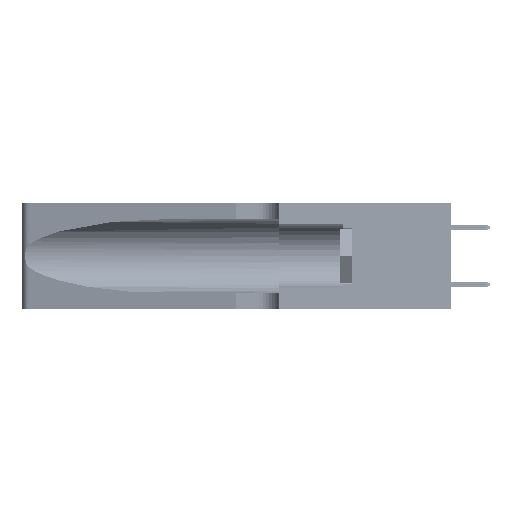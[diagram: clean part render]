
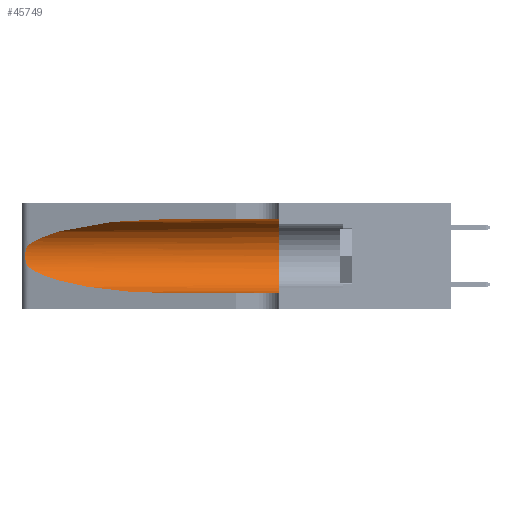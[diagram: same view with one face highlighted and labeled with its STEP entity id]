
A CAD part, left-side view. The second image highlights one B-rep face of the part: STEP entity #45749.
In plain terms, the highlighted cylindrical face has radius 3.308 mm (diameter 6.617 mm), a partial arc.
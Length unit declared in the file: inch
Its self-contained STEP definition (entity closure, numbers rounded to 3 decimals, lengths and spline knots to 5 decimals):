
#365 = CARTESIAN_POINT ( 'NONE',  ( 0.25487, 1.22718, 0.14631 ) ) ;
#1262 = CARTESIAN_POINT ( 'NONE',  ( 0.26075, 1.23896, 0.178 ) ) ;
#1339 = LINE ( 'NONE', #4804, #31778 ) ;
#3054 = CARTESIAN_POINT ( 'NONE',  ( 0.25487, 1.22718, 0.14631 ) ) ;
#4714 = AXIS2_PLACEMENT_3D ( 'NONE', #52521, #40748, #29009 ) ;
#4804 = CARTESIAN_POINT ( 'NONE',  ( 0.1305, 1.61858, 0.31525 ) ) ;
#5241 = CARTESIAN_POINT ( 'NONE',  ( 0.25854, 1.2359, 0.20912 ) ) ;
#7118 = CARTESIAN_POINT ( 'NONE',  ( 0.25487, 1.22718, 0.22369 ) ) ;
#8503 = ORIENTED_EDGE ( 'NONE', *, *, #50109, .T. ) ;
#9162 = CARTESIAN_POINT ( 'NONE',  ( 0.1305, 0.35, 0.31525 ) ) ;
#9496 = CARTESIAN_POINT ( 'NONE',  ( 0.25789, 1.23486, 0.15765 ) ) ;
#10034 = CARTESIAN_POINT ( 'NONE',  ( 0.25555, 1.22993, 0.14849 ) ) ;
#10321 = CARTESIAN_POINT ( 'NONE',  ( 0.1305, 0.72297, 0.31525 ) ) ;
#10965 = EDGE_CURVE ( 'NONE', #51271, #24128, #16492, .T. ) ;
#11076 = ORIENTED_EDGE ( 'NONE', *, *, #30904, .F. ) ;
#11129 = DIRECTION ( 'NONE',  ( 0., 0., 1. ) ) ;
#11803 = CARTESIAN_POINT ( 'NONE',  ( 0.18966, 0.96281, 0.05475 ) ) ;
#12203 = CARTESIAN_POINT ( 'NONE',  ( 0.25487, 1.22718, 0.22369 ) ) ;
#13523 = CARTESIAN_POINT ( 'NONE',  ( 0.25856, 1.23593, 0.16098 ) ) ;
#14235 = VECTOR ( 'NONE', #42158, 39.37008 ) ;
#14347 = CARTESIAN_POINT ( 'NONE',  ( 0.1305, 1.61858, 0.05475 ) ) ;
#14783 = EDGE_CURVE ( 'NONE', #21558, #20573, #14795, .T. ) ;
#14795 = CIRCLE ( 'NONE', #19038, 0.13025 ) ;
#15840 = ORIENTED_EDGE ( 'NONE', *, *, #45463, .T. ) ;
#16492 =( BOUNDED_CURVE ( )  B_SPLINE_CURVE ( 3, ( #3054, #31640, #11803, #37213 ),
 .UNSPECIFIED., .F., .F. ) 
 B_SPLINE_CURVE_WITH_KNOTS ( ( 4, 4 ),
 ( 3.44316, 4.71239 ),
 .UNSPECIFIED. ) 
 CURVE ( )  GEOMETRIC_REPRESENTATION_ITEM ( )  RATIONAL_B_SPLINE_CURVE ( ( 1., 0.87, 0.87, 1. ) ) 
 REPRESENTATION_ITEM ( '' )  );
#17354 = CARTESIAN_POINT ( 'NONE',  ( 0.1305, 0.72297, 0.31525 ) ) ;
#17631 = DIRECTION ( 'NONE',  ( 0., -1., 0. ) ) ;
#18364 = LINE ( 'NONE', #14347, #14235 ) ;
#18634 = CARTESIAN_POINT ( 'NONE',  ( 0.18966, 0.96281, 0.31525 ) ) ;
#19038 = AXIS2_PLACEMENT_3D ( 'NONE', #23740, #27726, #11129 ) ;
#19954 = CYLINDRICAL_SURFACE ( 'NONE', #4714, 0.13025 ) ;
#20275 = B_SPLINE_CURVE_WITH_KNOTS ( 'NONE', 3,
 ( #12203, #25594, #41873, #49886, #5241, #21577, #37866, #1262, #48826, #13523, #9496, #25859, #10034, #50384 ),
 .UNSPECIFIED., .F., .F.,
 ( 4, 2, 2, 2, 2, 2, 4 ),
 ( 0., 0.00027, 0.00053, 0.00107, 0.0016, 0.00187, 0.00214 ),
 .UNSPECIFIED. ) ;
#20353 = EDGE_LOOP ( 'NONE', ( #8503, #15840, #39663, #47136, #23297, #11076 ) ) ;
#20441 = VERTEX_POINT ( 'NONE', #25541 ) ;
#20573 = VERTEX_POINT ( 'NONE', #29908 ) ;
#21558 = VERTEX_POINT ( 'NONE', #9162 ) ;
#21577 = CARTESIAN_POINT ( 'NONE',  ( 0.26018, 1.23835, 0.19895 ) ) ;
#23297 = ORIENTED_EDGE ( 'NONE', *, *, #14783, .F. ) ;
#23740 = CARTESIAN_POINT ( 'NONE',  ( 0.1305, 0.35, 0.185 ) ) ;
#23971 = FACE_OUTER_BOUND ( 'NONE', #20353, .T. ) ;
#24128 = VERTEX_POINT ( 'NONE', #33075 ) ;
#25541 = CARTESIAN_POINT ( 'NONE',  ( 0.25487, 1.22718, 0.22369 ) ) ;
#25594 = CARTESIAN_POINT ( 'NONE',  ( 0.25555, 1.22994, 0.2215 ) ) ;
#25859 = CARTESIAN_POINT ( 'NONE',  ( 0.25639, 1.23186, 0.15144 ) ) ;
#27726 = DIRECTION ( 'NONE',  ( 0., 1., 0. ) ) ;
#29009 = DIRECTION ( 'NONE',  ( 0., 0., -1. ) ) ;
#29908 = CARTESIAN_POINT ( 'NONE',  ( 0.1305, 0.35, 0.05475 ) ) ;
#30904 = EDGE_CURVE ( 'NONE', #46910, #21558, #1339, .T. ) ;
#31640 = CARTESIAN_POINT ( 'NONE',  ( 0.2373, 1.15595, 0.08982 ) ) ;
#31778 = VECTOR ( 'NONE', #17631, 39.37008 ) ;
#33075 = CARTESIAN_POINT ( 'NONE',  ( 0.1305, 0.72297, 0.05475 ) ) ;
#34644 =( BOUNDED_CURVE ( )  B_SPLINE_CURVE ( 3, ( #10321, #18634, #51757, #7118 ),
 .UNSPECIFIED., .F., .T. ) 
 B_SPLINE_CURVE_WITH_KNOTS ( ( 4, 4 ),
 ( 1.5708, 2.84003 ),
 .UNSPECIFIED. ) 
 CURVE ( )  GEOMETRIC_REPRESENTATION_ITEM ( )  RATIONAL_B_SPLINE_CURVE ( ( 1., 0.87, 0.87, 1. ) ) 
 REPRESENTATION_ITEM ( '' )  );
#37213 = CARTESIAN_POINT ( 'NONE',  ( 0.1305, 0.72297, 0.05475 ) ) ;
#37866 = CARTESIAN_POINT ( 'NONE',  ( 0.26075, 1.23896, 0.19203 ) ) ;
#39663 = ORIENTED_EDGE ( 'NONE', *, *, #10965, .T. ) ;
#40748 = DIRECTION ( 'NONE',  ( 0., -1., 0. ) ) ;
#41873 = CARTESIAN_POINT ( 'NONE',  ( 0.25639, 1.23184, 0.21858 ) ) ;
#42158 = DIRECTION ( 'NONE',  ( 0., -1., 0. ) ) ;
#45463 = EDGE_CURVE ( 'NONE', #20441, #51271, #20275, .T. ) ;
#45749 = ADVANCED_FACE ( 'NONE', ( #23971 ), #19954, .F. ) ;
#46910 = VERTEX_POINT ( 'NONE', #17354 ) ;
#47136 = ORIENTED_EDGE ( 'NONE', *, *, #50392, .T. ) ;
#48826 = CARTESIAN_POINT ( 'NONE',  ( 0.26017, 1.23833, 0.17102 ) ) ;
#49886 = CARTESIAN_POINT ( 'NONE',  ( 0.25787, 1.23484, 0.2124 ) ) ;
#50109 = EDGE_CURVE ( 'NONE', #46910, #20441, #34644, .T. ) ;
#50384 = CARTESIAN_POINT ( 'NONE',  ( 0.25487, 1.22718, 0.14631 ) ) ;
#50392 = EDGE_CURVE ( 'NONE', #24128, #20573, #18364, .T. ) ;
#51271 = VERTEX_POINT ( 'NONE', #365 ) ;
#51757 = CARTESIAN_POINT ( 'NONE',  ( 0.2373, 1.15595, 0.28018 ) ) ;
#52521 = CARTESIAN_POINT ( 'NONE',  ( 0.1305, 1.61858, 0.185 ) ) ;
